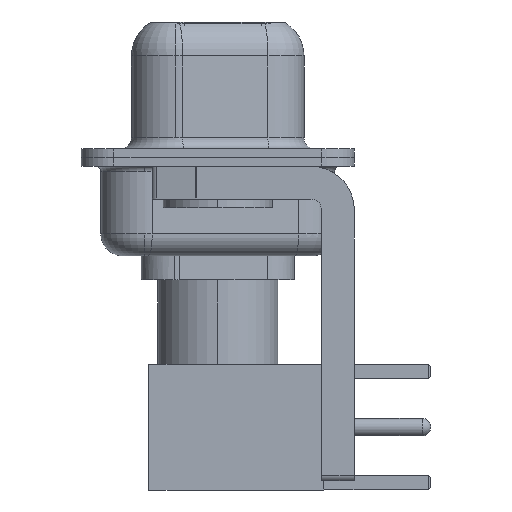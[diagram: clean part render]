
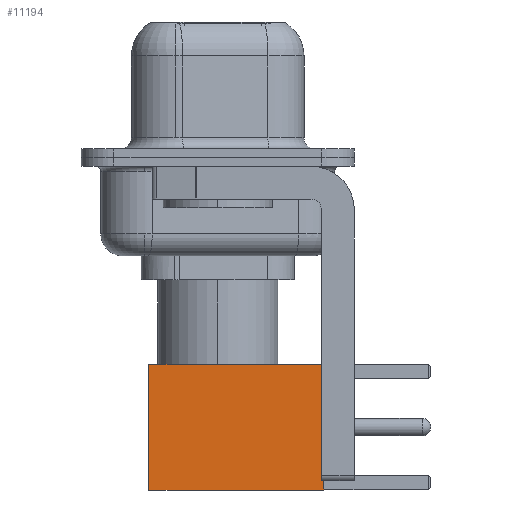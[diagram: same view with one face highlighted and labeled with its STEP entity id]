
A CAD part, left-side view. The second image highlights one B-rep face of the part: STEP entity #11194.
In plain terms, the highlighted face is planar.
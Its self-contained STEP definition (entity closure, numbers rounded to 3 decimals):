
#976 = VERTEX_POINT ( 'NONE', #6142 ) ;
#977 = PLANE ( 'NONE',  #14304 ) ;
#1145 = ORIENTED_EDGE ( 'NONE', *, *, #14258, .T. ) ;
#1344 = VECTOR ( 'NONE', #7036, 1000. ) ;
#1799 = ORIENTED_EDGE ( 'NONE', *, *, #9733, .F. ) ;
#2006 = EDGE_CURVE ( 'NONE', #8280, #6475, #11560, .T. ) ;
#2528 = CARTESIAN_POINT ( 'NONE',  ( 2.875, 2.875, 0. ) ) ;
#3111 = VECTOR ( 'NONE', #10568, 1000. ) ;
#3231 = LINE ( 'NONE', #4639, #1344 ) ;
#3317 = DIRECTION ( 'NONE',  ( 0., 1., 0. ) ) ;
#3766 = DIRECTION ( 'NONE',  ( 0., 0., -1. ) ) ;
#3865 = VERTEX_POINT ( 'NONE', #6278 ) ;
#3934 = CARTESIAN_POINT ( 'NONE',  ( -2.875, 2.875, 8. ) ) ;
#4639 = CARTESIAN_POINT ( 'NONE',  ( -2.875, 2.875, 0. ) ) ;
#5395 = VECTOR ( 'NONE', #3766, 1000. ) ;
#6142 = CARTESIAN_POINT ( 'NONE',  ( 2.875, 2.875, 0. ) ) ;
#6278 = CARTESIAN_POINT ( 'NONE',  ( -2.875, 2.875, 0. ) ) ;
#6475 = VERTEX_POINT ( 'NONE', #3934 ) ;
#7027 = LINE ( 'NONE', #13118, #3111 ) ;
#7036 = DIRECTION ( 'NONE',  ( 0., 0., -1. ) ) ;
#8280 = VERTEX_POINT ( 'NONE', #15437 ) ;
#8346 = DIRECTION ( 'NONE',  ( 0., 0., 1. ) ) ;
#9578 = CARTESIAN_POINT ( 'NONE',  ( 2.875, 2.875, 0. ) ) ;
#9733 = EDGE_CURVE ( 'NONE', #6475, #3865, #3231, .T. ) ;
#10228 = EDGE_LOOP ( 'NONE', ( #1145, #11772, #1799, #10539 ) ) ;
#10404 = CARTESIAN_POINT ( 'NONE',  ( 0., 2.875, 8. ) ) ;
#10539 = ORIENTED_EDGE ( 'NONE', *, *, #2006, .F. ) ;
#10568 = DIRECTION ( 'NONE',  ( -1., 0., 0. ) ) ;
#11194 = ADVANCED_FACE ( 'NONE', ( #14768 ), #977, .T. ) ;
#11560 = LINE ( 'NONE', #10404, #13286 ) ;
#11772 = ORIENTED_EDGE ( 'NONE', *, *, #15499, .T. ) ;
#13118 = CARTESIAN_POINT ( 'NONE',  ( 0., 2.875, 0. ) ) ;
#13286 = VECTOR ( 'NONE', #15199, 1000. ) ;
#14258 = EDGE_CURVE ( 'NONE', #8280, #976, #16236, .T. ) ;
#14304 = AXIS2_PLACEMENT_3D ( 'NONE', #9578, #3317, #8346 ) ;
#14768 = FACE_OUTER_BOUND ( 'NONE', #10228, .T. ) ;
#15199 = DIRECTION ( 'NONE',  ( -1., 0., 0. ) ) ;
#15437 = CARTESIAN_POINT ( 'NONE',  ( 2.875, 2.875, 8. ) ) ;
#15499 = EDGE_CURVE ( 'NONE', #976, #3865, #7027, .T. ) ;
#16236 = LINE ( 'NONE', #2528, #5395 ) ;
